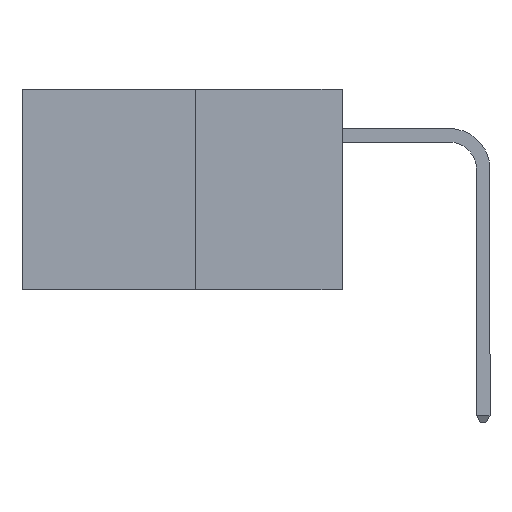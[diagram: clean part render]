
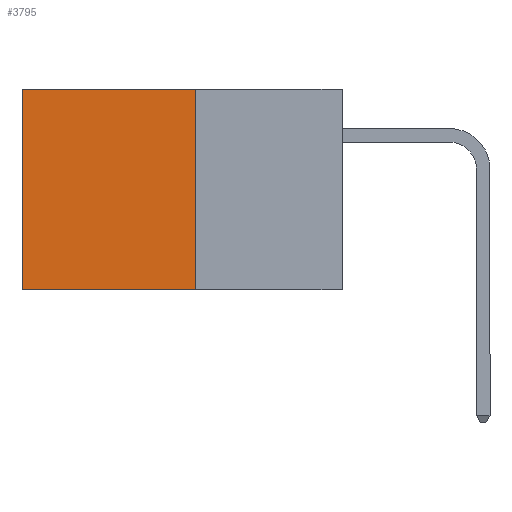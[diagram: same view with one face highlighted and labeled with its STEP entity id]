
A CAD part, left-side view. The second image highlights one B-rep face of the part: STEP entity #3795.
In plain terms, the highlighted planar face has unit normal (-1, 0, 0).
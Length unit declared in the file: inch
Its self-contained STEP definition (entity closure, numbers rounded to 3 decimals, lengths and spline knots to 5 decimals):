
#359 = CARTESIAN_POINT ( 'NONE',  ( 0.277, 0.27, 0. ) ) ;
#474 = CARTESIAN_POINT ( 'NONE',  ( 0.277, 0.59, -0.37 ) ) ;
#637 = VECTOR ( 'NONE', #6410, 39.37008 ) ;
#830 = VERTEX_POINT ( 'NONE', #5746 ) ;
#1246 = LINE ( 'NONE', #6188, #8622 ) ;
#2067 = EDGE_CURVE ( 'NONE', #3920, #830, #3939, .T. ) ;
#2097 = VECTOR ( 'NONE', #2798, 39.37008 ) ;
#2174 = VECTOR ( 'NONE', #4854, 39.37008 ) ;
#2561 = LINE ( 'NONE', #2731, #2097 ) ;
#2731 = CARTESIAN_POINT ( 'NONE',  ( 0.277, 0.27, 0. ) ) ;
#2798 = DIRECTION ( 'NONE',  ( 0., 1., 0. ) ) ;
#2937 = CARTESIAN_POINT ( 'NONE',  ( 0.277, 0.27, -0.37 ) ) ;
#3795 = ADVANCED_FACE ( 'NONE', ( #6054 ), #4616, .F. ) ;
#3920 = VERTEX_POINT ( 'NONE', #359 ) ;
#3939 = LINE ( 'NONE', #4832, #2174 ) ;
#4042 = DIRECTION ( 'NONE',  ( 0., 0., -1. ) ) ;
#4093 = DIRECTION ( 'NONE',  ( 1., 0., 0. ) ) ;
#4616 = PLANE ( 'NONE',  #6533 ) ;
#4633 = VERTEX_POINT ( 'NONE', #474 ) ;
#4832 = CARTESIAN_POINT ( 'NONE',  ( 0.277, 0.27, -0.37 ) ) ;
#4854 = DIRECTION ( 'NONE',  ( 0., 0., -1. ) ) ;
#5655 = ORIENTED_EDGE ( 'NONE', *, *, #6710, .F. ) ;
#5746 = CARTESIAN_POINT ( 'NONE',  ( 0.277, 0.27, -0.37 ) ) ;
#6054 = FACE_OUTER_BOUND ( 'NONE', #7694, .T. ) ;
#6188 = CARTESIAN_POINT ( 'NONE',  ( 0.277, 0.59, -0.37 ) ) ;
#6410 = DIRECTION ( 'NONE',  ( 0., 1., 0. ) ) ;
#6533 = AXIS2_PLACEMENT_3D ( 'NONE', #7006, #4093, #4042 ) ;
#6710 = EDGE_CURVE ( 'NONE', #830, #4633, #8764, .T. ) ;
#6945 = DIRECTION ( 'NONE',  ( 0., 0., -1. ) ) ;
#7006 = CARTESIAN_POINT ( 'NONE',  ( 0.277, 0.27, -0.37 ) ) ;
#7162 = ORIENTED_EDGE ( 'NONE', *, *, #9424, .T. ) ;
#7604 = ORIENTED_EDGE ( 'NONE', *, *, #2067, .F. ) ;
#7694 = EDGE_LOOP ( 'NONE', ( #7162, #5655, #7604, #8245 ) ) ;
#8208 = EDGE_CURVE ( 'NONE', #3920, #8646, #2561, .T. ) ;
#8245 = ORIENTED_EDGE ( 'NONE', *, *, #8208, .T. ) ;
#8622 = VECTOR ( 'NONE', #6945, 39.37008 ) ;
#8646 = VERTEX_POINT ( 'NONE', #9371 ) ;
#8764 = LINE ( 'NONE', #2937, #637 ) ;
#9371 = CARTESIAN_POINT ( 'NONE',  ( 0.277, 0.59, 0. ) ) ;
#9424 = EDGE_CURVE ( 'NONE', #8646, #4633, #1246, .T. ) ;
